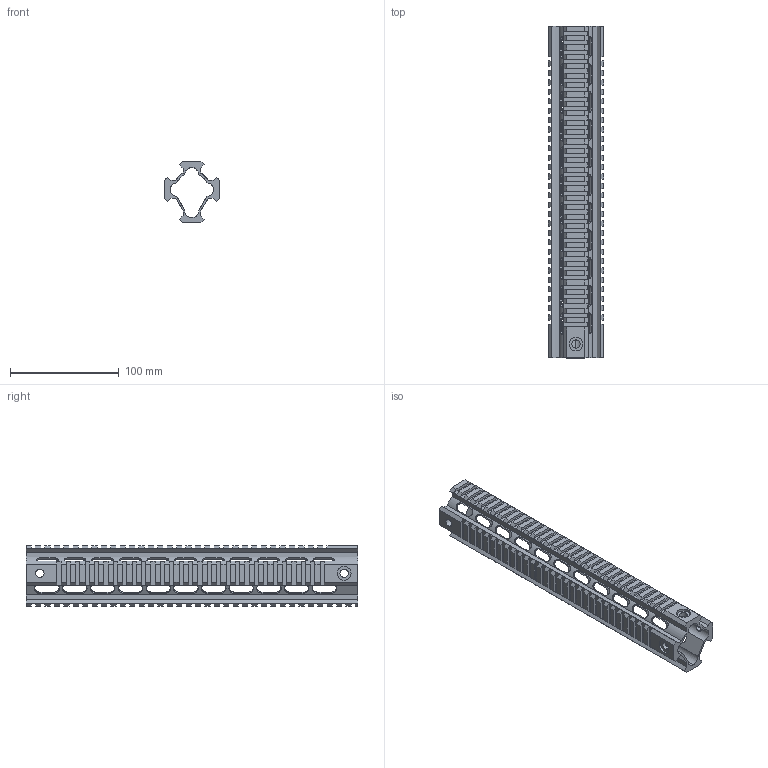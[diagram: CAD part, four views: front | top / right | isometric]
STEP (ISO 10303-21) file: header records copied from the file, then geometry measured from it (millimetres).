
FILE_DESCRIPTION (( 'STEP AP214' ), '1' );
FILE_NAME ('quad-rail-hand-guard.STEP', '2013-05-23T13:43:56', ( 'Asher' ), ( '' ), 'SwSTEP 2.0', 'SolidWorks 2013', '' );
FILE_SCHEMA (( 'AUTOMOTIVE_DESIGN' ));
Length unit declared in the file: inch
Products named in the file (1): quad-rail-hand-guard
Bounding box: 50.8 x 304.8 x 55.74 mm (x, y, z)
Volume: 160657.3 mm3; surface area: 108507.2 mm2
Topology: 1 solids, 1 shells, 738 faces, 2199 edges, 1466 vertices
Faces by surface type: plane 625, cylinder 113
Entity records: 37121 total; most frequent: CARTESIAN_POINT 7692, ORIENTED_EDGE 4398, DIRECTION 3619, EDGE_CURVE 2199, LINE 1973, VECTOR 1973, VERTEX_POINT 1466, EDGE_LOOP 841
